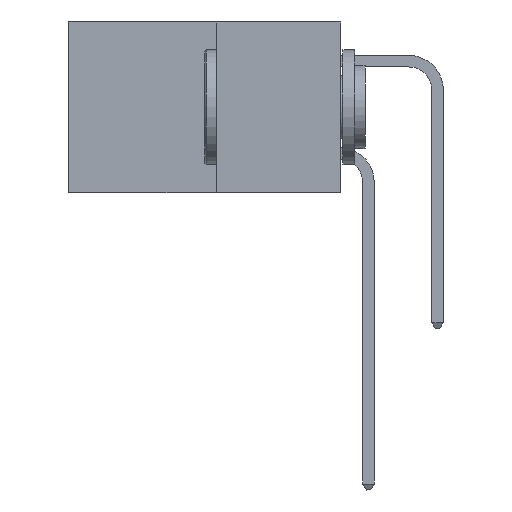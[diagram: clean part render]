
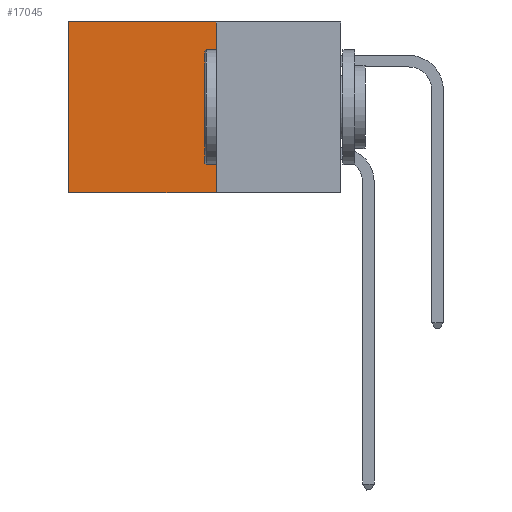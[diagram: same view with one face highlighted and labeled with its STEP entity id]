
A CAD part, left-side view. The second image highlights one B-rep face of the part: STEP entity #17045.
In plain terms, the highlighted planar face has unit normal (-1, 0, 0).
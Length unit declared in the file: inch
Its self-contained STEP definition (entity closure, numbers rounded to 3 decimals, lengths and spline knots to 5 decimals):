
#563 = EDGE_CURVE ( 'NONE', #12152, #11648, #19740, .T. ) ;
#748 = CARTESIAN_POINT ( 'NONE',  ( 0.277, 0.59, -0.37 ) ) ;
#951 = LINE ( 'NONE', #1748, #15155 ) ;
#1748 = CARTESIAN_POINT ( 'NONE',  ( 0.277, 0.59, -0.37 ) ) ;
#4250 = CARTESIAN_POINT ( 'NONE',  ( 0.277, 0.27, 0. ) ) ;
#4374 = VERTEX_POINT ( 'NONE', #748 ) ;
#4759 = ORIENTED_EDGE ( 'NONE', *, *, #25195, .F. ) ;
#6293 = CARTESIAN_POINT ( 'NONE',  ( 0.277, 0.27, -0.37 ) ) ;
#7095 = ORIENTED_EDGE ( 'NONE', *, *, #563, .T. ) ;
#7633 = DIRECTION ( 'NONE',  ( 0., 1., 0. ) ) ;
#7646 = EDGE_CURVE ( 'NONE', #12598, #4374, #31539, .T. ) ;
#10146 = CARTESIAN_POINT ( 'NONE',  ( 0.277, 0.27, -0.37 ) ) ;
#11643 = CARTESIAN_POINT ( 'NONE',  ( 0.277, 0.27, -0.37 ) ) ;
#11648 = VERTEX_POINT ( 'NONE', #15538 ) ;
#12152 = VERTEX_POINT ( 'NONE', #4250 ) ;
#12598 = VERTEX_POINT ( 'NONE', #28061 ) ;
#13365 = VECTOR ( 'NONE', #7633, 39.37008 ) ;
#14021 = EDGE_CURVE ( 'NONE', #11648, #4374, #951, .T. ) ;
#14468 = DIRECTION ( 'NONE',  ( 0., 1., 0. ) ) ;
#14855 = DIRECTION ( 'NONE',  ( 1., 0., 0. ) ) ;
#15155 = VECTOR ( 'NONE', #34604, 39.37008 ) ;
#15538 = CARTESIAN_POINT ( 'NONE',  ( 0.277, 0.59, 0. ) ) ;
#16010 = ORIENTED_EDGE ( 'NONE', *, *, #14021, .T. ) ;
#17009 = EDGE_LOOP ( 'NONE', ( #16010, #35432, #4759, #7095 ) ) ;
#17045 = ADVANCED_FACE ( 'NONE', ( #35398 ), #30950, .F. ) ;
#19617 = VECTOR ( 'NONE', #23778, 39.37008 ) ;
#19740 = LINE ( 'NONE', #30180, #13365 ) ;
#23778 = DIRECTION ( 'NONE',  ( 0., 0., -1. ) ) ;
#24454 = VECTOR ( 'NONE', #14468, 39.37008 ) ;
#25195 = EDGE_CURVE ( 'NONE', #12152, #12598, #26814, .T. ) ;
#26814 = LINE ( 'NONE', #10146, #19617 ) ;
#28061 = CARTESIAN_POINT ( 'NONE',  ( 0.277, 0.27, -0.37 ) ) ;
#29394 = AXIS2_PLACEMENT_3D ( 'NONE', #6293, #14855, #33615 ) ;
#30180 = CARTESIAN_POINT ( 'NONE',  ( 0.277, 0.27, 0. ) ) ;
#30950 = PLANE ( 'NONE',  #29394 ) ;
#31539 = LINE ( 'NONE', #11643, #24454 ) ;
#33615 = DIRECTION ( 'NONE',  ( 0., 0., -1. ) ) ;
#34604 = DIRECTION ( 'NONE',  ( 0., 0., -1. ) ) ;
#35398 = FACE_OUTER_BOUND ( 'NONE', #17009, .T. ) ;
#35432 = ORIENTED_EDGE ( 'NONE', *, *, #7646, .F. ) ;
